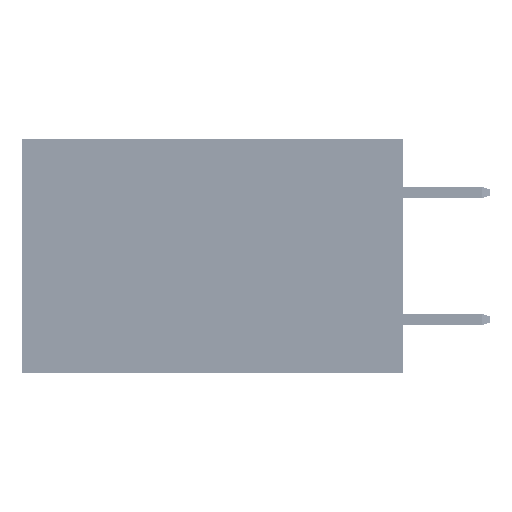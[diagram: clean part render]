
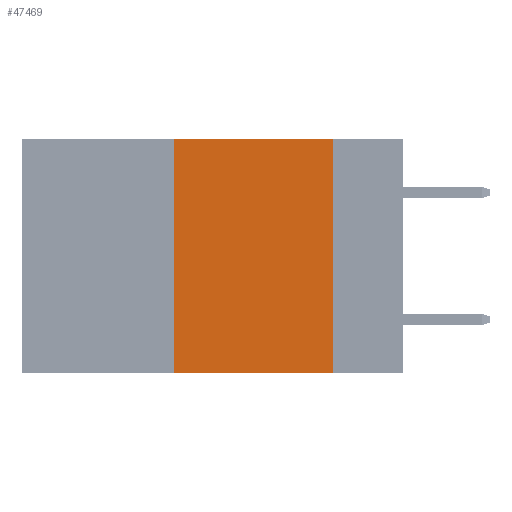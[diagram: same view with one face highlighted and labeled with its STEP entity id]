
A CAD part, left-side view. The second image highlights one B-rep face of the part: STEP entity #47469.
In plain terms, the highlighted planar face has unit normal (-1, 0, 0).
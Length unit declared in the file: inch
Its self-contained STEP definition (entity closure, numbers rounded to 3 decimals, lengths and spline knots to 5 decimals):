
#739 = EDGE_LOOP ( 'NONE', ( #2436, #18041, #18145, #31475 ) ) ;
#1359 = EDGE_CURVE ( 'NONE', #2311, #5903, #15087, .T. ) ;
#2311 = VERTEX_POINT ( 'NONE', #10498 ) ;
#2436 = ORIENTED_EDGE ( 'NONE', *, *, #9768, .F. ) ;
#3163 = LINE ( 'NONE', #18969, #11655 ) ;
#3430 = CARTESIAN_POINT ( 'NONE',  ( 0., 0.11, 0. ) ) ;
#5333 = PLANE ( 'NONE',  #46083 ) ;
#5726 = EDGE_CURVE ( 'NONE', #2311, #36583, #3163, .T. ) ;
#5903 = VERTEX_POINT ( 'NONE', #12625 ) ;
#6492 = LINE ( 'NONE', #49783, #18134 ) ;
#9768 = EDGE_CURVE ( 'NONE', #43769, #5903, #15535, .T. ) ;
#10498 = CARTESIAN_POINT ( 'NONE',  ( 0., 0.36, -0.37 ) ) ;
#11341 = DIRECTION ( 'NONE',  ( 0., 0., -1. ) ) ;
#11655 = VECTOR ( 'NONE', #23460, 39.37008 ) ;
#12625 = CARTESIAN_POINT ( 'NONE',  ( 0., 0.11, -0.37 ) ) ;
#12673 = CARTESIAN_POINT ( 'NONE',  ( 0., 0.36, 0. ) ) ;
#15087 = LINE ( 'NONE', #30387, #51404 ) ;
#15535 = LINE ( 'NONE', #3430, #42208 ) ;
#18041 = ORIENTED_EDGE ( 'NONE', *, *, #37387, .F. ) ;
#18134 = VECTOR ( 'NONE', #29250, 39.37008 ) ;
#18145 = ORIENTED_EDGE ( 'NONE', *, *, #5726, .F. ) ;
#18969 = CARTESIAN_POINT ( 'NONE',  ( 0., 0.36, 0. ) ) ;
#23460 = DIRECTION ( 'NONE',  ( 0., 0., 1. ) ) ;
#26947 = CARTESIAN_POINT ( 'NONE',  ( 0., 0.11, 0. ) ) ;
#29250 = DIRECTION ( 'NONE',  ( 0., -1., 0. ) ) ;
#29324 = DIRECTION ( 'NONE',  ( 1., 0., 0. ) ) ;
#30387 = CARTESIAN_POINT ( 'NONE',  ( 0., 0.6, -0.37 ) ) ;
#31475 = ORIENTED_EDGE ( 'NONE', *, *, #1359, .T. ) ;
#36583 = VERTEX_POINT ( 'NONE', #12673 ) ;
#37387 = EDGE_CURVE ( 'NONE', #36583, #43769, #6492, .T. ) ;
#37999 = DIRECTION ( 'NONE',  ( 0., 0., -1. ) ) ;
#41183 = CARTESIAN_POINT ( 'NONE',  ( 0., 0.6, 0. ) ) ;
#42208 = VECTOR ( 'NONE', #11341, 39.37008 ) ;
#43769 = VERTEX_POINT ( 'NONE', #26947 ) ;
#46083 = AXIS2_PLACEMENT_3D ( 'NONE', #41183, #29324, #37999 ) ;
#46171 = FACE_OUTER_BOUND ( 'NONE', #739, .T. ) ;
#46472 = DIRECTION ( 'NONE',  ( 0., -1., 0. ) ) ;
#47469 = ADVANCED_FACE ( 'NONE', ( #46171 ), #5333, .F. ) ;
#49783 = CARTESIAN_POINT ( 'NONE',  ( 0., 0.6, 0. ) ) ;
#51404 = VECTOR ( 'NONE', #46472, 39.37008 ) ;
